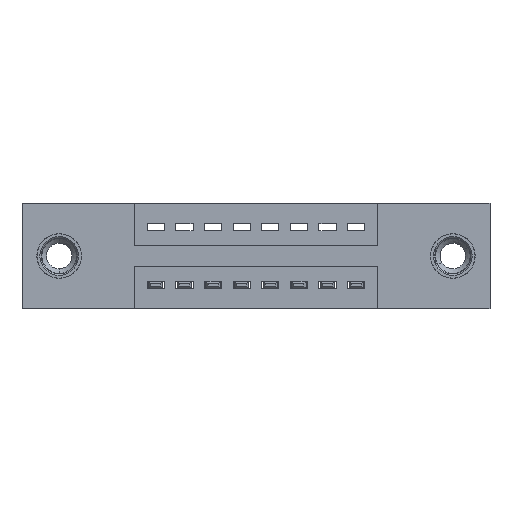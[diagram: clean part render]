
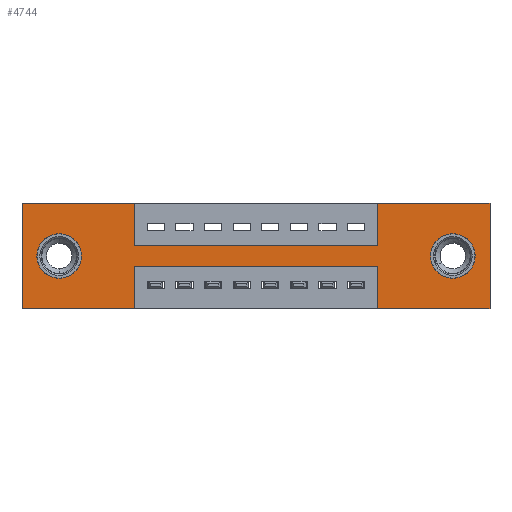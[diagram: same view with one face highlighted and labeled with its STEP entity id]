
A CAD part, front view. The second image highlights one B-rep face of the part: STEP entity #4744.
In plain terms, the highlighted planar face has unit normal (0, -1, 0).
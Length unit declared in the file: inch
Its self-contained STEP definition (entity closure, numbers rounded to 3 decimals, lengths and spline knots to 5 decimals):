
#79 = AXIS2_PLACEMENT_3D ( 'NONE', #8976, #5361, #6257 ) ;
#159 = ORIENTED_EDGE ( 'NONE', *, *, #9862, .T. ) ;
#173 = EDGE_CURVE ( 'NONE', #3503, #5836, #4946, .T. ) ;
#188 = VERTEX_POINT ( 'NONE', #8156 ) ;
#208 = CARTESIAN_POINT ( 'NONE',  ( 1.505, 0., -0.107 ) ) ;
#223 = VERTEX_POINT ( 'NONE', #10902 ) ;
#288 = VERTEX_POINT ( 'NONE', #9231 ) ;
#300 = FACE_BOUND ( 'NONE', #9448, .T. ) ;
#363 = VERTEX_POINT ( 'NONE', #1614 ) ;
#659 = CIRCLE ( 'NONE', #1015, 0.078 ) ;
#731 = VERTEX_POINT ( 'NONE', #208 ) ;
#736 = EDGE_CURVE ( 'NONE', #2956, #188, #1029, .T. ) ;
#751 = LINE ( 'NONE', #8270, #7325 ) ;
#912 = DIRECTION ( 'NONE',  ( 0., 0., 1. ) ) ;
#1005 = VERTEX_POINT ( 'NONE', #4444 ) ;
#1015 = AXIS2_PLACEMENT_3D ( 'NONE', #9903, #4414, #912 ) ;
#1029 = LINE ( 'NONE', #9124, #4247 ) ;
#1494 = CARTESIAN_POINT ( 'NONE',  ( 0., 0., 0. ) ) ;
#1502 = EDGE_CURVE ( 'NONE', #1005, #6854, #659, .T. ) ;
#1598 = ORIENTED_EDGE ( 'NONE', *, *, #11032, .F. ) ;
#1612 = ORIENTED_EDGE ( 'NONE', *, *, #1502, .T. ) ;
#1614 = CARTESIAN_POINT ( 'NONE',  ( 1.2425, 0., -0.22 ) ) ;
#1804 = ORIENTED_EDGE ( 'NONE', *, *, #6903, .T. ) ;
#1862 = CARTESIAN_POINT ( 'NONE',  ( 0., 0., -0.37 ) ) ;
#2054 = EDGE_CURVE ( 'NONE', #4793, #2956, #10048, .T. ) ;
#2166 = VECTOR ( 'NONE', #6839, 39.37008 ) ;
#2181 = EDGE_CURVE ( 'NONE', #223, #7047, #4538, .T. ) ;
#2402 = CARTESIAN_POINT ( 'NONE',  ( 0.3925, 0., 0. ) ) ;
#2825 = VECTOR ( 'NONE', #11174, 39.37008 ) ;
#2863 = DIRECTION ( 'NONE',  ( 0., 0., -1. ) ) ;
#2956 = VERTEX_POINT ( 'NONE', #8385 ) ;
#2975 = LINE ( 'NONE', #10501, #11419 ) ;
#2992 = LINE ( 'NONE', #7980, #6350 ) ;
#2996 = ORIENTED_EDGE ( 'NONE', *, *, #2054, .F. ) ;
#3019 = CARTESIAN_POINT ( 'NONE',  ( 0., 0., -0.37 ) ) ;
#3260 = CARTESIAN_POINT ( 'NONE',  ( 0.13, 0., -0.185 ) ) ;
#3354 = ORIENTED_EDGE ( 'NONE', *, *, #3640, .F. ) ;
#3400 = ORIENTED_EDGE ( 'NONE', *, *, #736, .F. ) ;
#3503 = VERTEX_POINT ( 'NONE', #6025 ) ;
#3640 = EDGE_CURVE ( 'NONE', #7907, #3503, #2975, .T. ) ;
#3734 = EDGE_CURVE ( 'NONE', #288, #731, #9870, .T. ) ;
#3758 = EDGE_CURVE ( 'NONE', #6385, #4793, #6197, .T. ) ;
#3793 = DIRECTION ( 'NONE',  ( 0., 0., 1. ) ) ;
#4068 = FACE_OUTER_BOUND ( 'NONE', #9574, .T. ) ;
#4139 = DIRECTION ( 'NONE',  ( 0., -1., 0. ) ) ;
#4247 = VECTOR ( 'NONE', #10781, 39.37008 ) ;
#4255 = AXIS2_PLACEMENT_3D ( 'NONE', #5718, #4139, #8623 ) ;
#4284 = ORIENTED_EDGE ( 'NONE', *, *, #2181, .F. ) ;
#4305 = DIRECTION ( 'NONE',  ( 0., 1., 0. ) ) ;
#4414 = DIRECTION ( 'NONE',  ( 0., 1., 0. ) ) ;
#4444 = CARTESIAN_POINT ( 'NONE',  ( 0.13, 0., -0.107 ) ) ;
#4459 = CARTESIAN_POINT ( 'NONE',  ( 0.13, 0., -0.263 ) ) ;
#4538 = LINE ( 'NONE', #8122, #7656 ) ;
#4643 = CARTESIAN_POINT ( 'NONE',  ( 1.2425, 0., 0. ) ) ;
#4702 = CARTESIAN_POINT ( 'NONE',  ( 0., 0., 0. ) ) ;
#4726 = PLANE ( 'NONE',  #4255 ) ;
#4744 = ADVANCED_FACE ( 'NONE', ( #300, #6050, #4068 ), #4726, .T. ) ;
#4793 = VERTEX_POINT ( 'NONE', #6777 ) ;
#4797 = VERTEX_POINT ( 'NONE', #1494 ) ;
#4946 = LINE ( 'NONE', #1862, #9184 ) ;
#5072 = AXIS2_PLACEMENT_3D ( 'NONE', #7347, #8266, #2863 ) ;
#5110 = VECTOR ( 'NONE', #7000, 39.37008 ) ;
#5120 = CIRCLE ( 'NONE', #11151, 0.078 ) ;
#5328 = VERTEX_POINT ( 'NONE', #2402 ) ;
#5361 = DIRECTION ( 'NONE',  ( 0., 1., 0. ) ) ;
#5419 = DIRECTION ( 'NONE',  ( 1., 0., 0. ) ) ;
#5718 = CARTESIAN_POINT ( 'NONE',  ( 0., 0., -0.37 ) ) ;
#5801 = LINE ( 'NONE', #9525, #2166 ) ;
#5836 = VERTEX_POINT ( 'NONE', #3019 ) ;
#5973 = ORIENTED_EDGE ( 'NONE', *, *, #10895, .F. ) ;
#6025 = CARTESIAN_POINT ( 'NONE',  ( 0.3925, 0., -0.37 ) ) ;
#6050 = FACE_BOUND ( 'NONE', #6510, .T. ) ;
#6194 = VECTOR ( 'NONE', #8359, 39.37008 ) ;
#6197 = LINE ( 'NONE', #4702, #2825 ) ;
#6252 = CIRCLE ( 'NONE', #79, 0.078 ) ;
#6257 = DIRECTION ( 'NONE',  ( 0., 0., -1. ) ) ;
#6328 = LINE ( 'NONE', #10275, #10979 ) ;
#6350 = VECTOR ( 'NONE', #8680, 39.37008 ) ;
#6385 = VERTEX_POINT ( 'NONE', #4643 ) ;
#6510 = EDGE_LOOP ( 'NONE', ( #1612, #159 ) ) ;
#6547 = CARTESIAN_POINT ( 'NONE',  ( 0., 0., 0. ) ) ;
#6777 = CARTESIAN_POINT ( 'NONE',  ( 1.635, 0., 0. ) ) ;
#6839 = DIRECTION ( 'NONE',  ( 0., 0., 1. ) ) ;
#6854 = VERTEX_POINT ( 'NONE', #4459 ) ;
#6903 = EDGE_CURVE ( 'NONE', #731, #288, #6252, .T. ) ;
#6914 = LINE ( 'NONE', #6547, #6194 ) ;
#6991 = DIRECTION ( 'NONE',  ( 0., 0., 1. ) ) ;
#6996 = CARTESIAN_POINT ( 'NONE',  ( 0.3925, 0., -0.22 ) ) ;
#7000 = DIRECTION ( 'NONE',  ( 0., 0., -1. ) ) ;
#7047 = VERTEX_POINT ( 'NONE', #10828 ) ;
#7158 = ORIENTED_EDGE ( 'NONE', *, *, #3758, .F. ) ;
#7170 = ORIENTED_EDGE ( 'NONE', *, *, #10115, .F. ) ;
#7243 = ORIENTED_EDGE ( 'NONE', *, *, #3734, .T. ) ;
#7325 = VECTOR ( 'NONE', #10807, 39.37008 ) ;
#7347 = CARTESIAN_POINT ( 'NONE',  ( 1.505, 0., -0.185 ) ) ;
#7478 = ORIENTED_EDGE ( 'NONE', *, *, #9924, .F. ) ;
#7656 = VECTOR ( 'NONE', #5419, 39.37008 ) ;
#7907 = VERTEX_POINT ( 'NONE', #10894 ) ;
#7980 = CARTESIAN_POINT ( 'NONE',  ( 0., 0., 0. ) ) ;
#8122 = CARTESIAN_POINT ( 'NONE',  ( 0.3925, 0., -0.15 ) ) ;
#8156 = CARTESIAN_POINT ( 'NONE',  ( 1.2425, 0., -0.37 ) ) ;
#8212 = LINE ( 'NONE', #6996, #8366 ) ;
#8266 = DIRECTION ( 'NONE',  ( 0., 1., 0. ) ) ;
#8270 = CARTESIAN_POINT ( 'NONE',  ( 0.3925, 0., 0. ) ) ;
#8309 = ORIENTED_EDGE ( 'NONE', *, *, #11091, .F. ) ;
#8359 = DIRECTION ( 'NONE',  ( 0., 0., 1. ) ) ;
#8366 = VECTOR ( 'NONE', #10618, 39.37008 ) ;
#8385 = CARTESIAN_POINT ( 'NONE',  ( 1.635, 0., -0.37 ) ) ;
#8533 = ORIENTED_EDGE ( 'NONE', *, *, #10055, .F. ) ;
#8623 = DIRECTION ( 'NONE',  ( 0., 0., -1. ) ) ;
#8680 = DIRECTION ( 'NONE',  ( 1., 0., 0. ) ) ;
#8976 = CARTESIAN_POINT ( 'NONE',  ( 1.505, 0., -0.185 ) ) ;
#9124 = CARTESIAN_POINT ( 'NONE',  ( 0., 0., -0.37 ) ) ;
#9184 = VECTOR ( 'NONE', #9886, 39.37008 ) ;
#9221 = DIRECTION ( 'NONE',  ( 0., 0., -1. ) ) ;
#9231 = CARTESIAN_POINT ( 'NONE',  ( 1.505, 0., -0.263 ) ) ;
#9448 = EDGE_LOOP ( 'NONE', ( #1804, #7243 ) ) ;
#9525 = CARTESIAN_POINT ( 'NONE',  ( 1.2425, 0., -0.37 ) ) ;
#9574 = EDGE_LOOP ( 'NONE', ( #3354, #7170, #8533, #3400, #2996, #7158, #8309, #4284, #5973, #7478, #1598, #9891 ) ) ;
#9654 = CARTESIAN_POINT ( 'NONE',  ( 1.635, 0., 0. ) ) ;
#9862 = EDGE_CURVE ( 'NONE', #6854, #1005, #5120, .T. ) ;
#9870 = CIRCLE ( 'NONE', #5072, 0.078 ) ;
#9886 = DIRECTION ( 'NONE',  ( -1., 0., 0. ) ) ;
#9891 = ORIENTED_EDGE ( 'NONE', *, *, #173, .F. ) ;
#9903 = CARTESIAN_POINT ( 'NONE',  ( 0.13, 0., -0.185 ) ) ;
#9924 = EDGE_CURVE ( 'NONE', #4797, #5328, #2992, .T. ) ;
#10048 = LINE ( 'NONE', #9654, #5110 ) ;
#10055 = EDGE_CURVE ( 'NONE', #188, #363, #5801, .T. ) ;
#10115 = EDGE_CURVE ( 'NONE', #363, #7907, #8212, .T. ) ;
#10275 = CARTESIAN_POINT ( 'NONE',  ( 1.2425, 0., 0. ) ) ;
#10501 = CARTESIAN_POINT ( 'NONE',  ( 0.3925, 0., -0.37 ) ) ;
#10618 = DIRECTION ( 'NONE',  ( -1., 0., 0. ) ) ;
#10781 = DIRECTION ( 'NONE',  ( -1., 0., 0. ) ) ;
#10807 = DIRECTION ( 'NONE',  ( 0., 0., -1. ) ) ;
#10828 = CARTESIAN_POINT ( 'NONE',  ( 1.2425, 0., -0.15 ) ) ;
#10894 = CARTESIAN_POINT ( 'NONE',  ( 0.3925, 0., -0.22 ) ) ;
#10895 = EDGE_CURVE ( 'NONE', #5328, #223, #751, .T. ) ;
#10902 = CARTESIAN_POINT ( 'NONE',  ( 0.3925, 0., -0.15 ) ) ;
#10979 = VECTOR ( 'NONE', #3793, 39.37008 ) ;
#11032 = EDGE_CURVE ( 'NONE', #5836, #4797, #6914, .T. ) ;
#11091 = EDGE_CURVE ( 'NONE', #7047, #6385, #6328, .T. ) ;
#11151 = AXIS2_PLACEMENT_3D ( 'NONE', #3260, #4305, #6991 ) ;
#11174 = DIRECTION ( 'NONE',  ( 1., 0., 0. ) ) ;
#11419 = VECTOR ( 'NONE', #9221, 39.37008 ) ;
